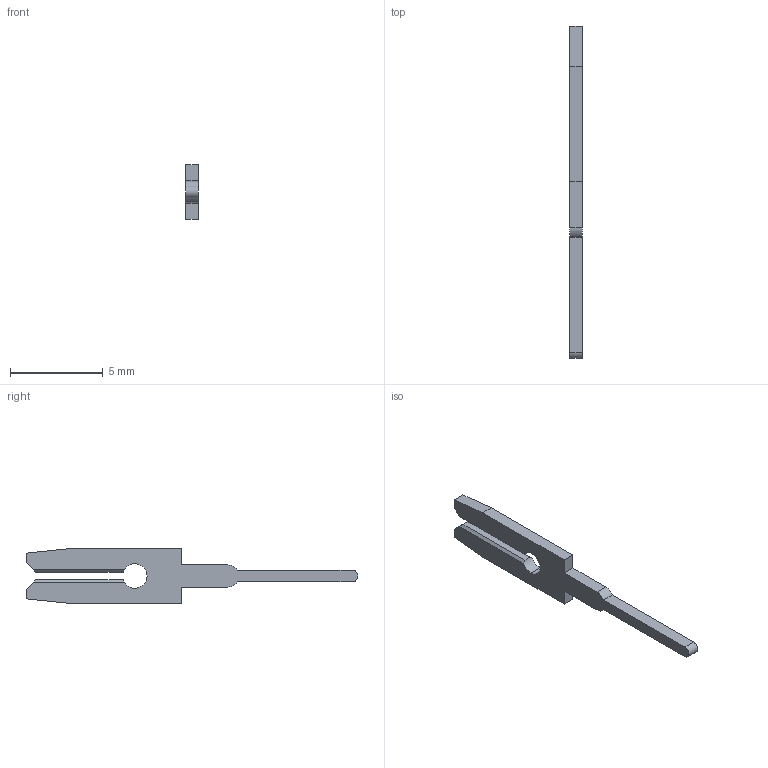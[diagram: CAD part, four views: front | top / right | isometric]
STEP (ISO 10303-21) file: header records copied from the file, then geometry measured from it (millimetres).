
FILE_DESCRIPTION (( 'STEP AP203' ), '1' );
FILE_NAME ('100-290-251.STEP', '2020-04-07T15:17:17', ( '' ), ( '' ), 'SwSTEP 2.0', 'SolidWorks 2016', '' );
FILE_SCHEMA (( 'CONFIG_CONTROL_DESIGN' ));
Length unit declared in the file: millimetre
Products named in the file (2): 100-290-251; 100-290-001_100-290-251
Assembly tree (1 placements, depth 2):
  100-290-251
    100-290-001_100-290-251
Bounding box: 0.66 x 17.91 x 2.92 mm (x, y, z)
Volume: 18.3 mm3; surface area: 89.9 mm2
Topology: 1 solids, 1 shells, 28 faces, 78 edges, 52 vertices
Faces by surface type: plane 22, cylinder 6
Entity records: 1090 total; most frequent: CARTESIAN_POINT 174, ORIENTED_EDGE 156, DIRECTION 150, EDGE_CURVE 78, LINE 62, VECTOR 62, VERTEX_POINT 52, AXIS2_PLACEMENT_3D 44
